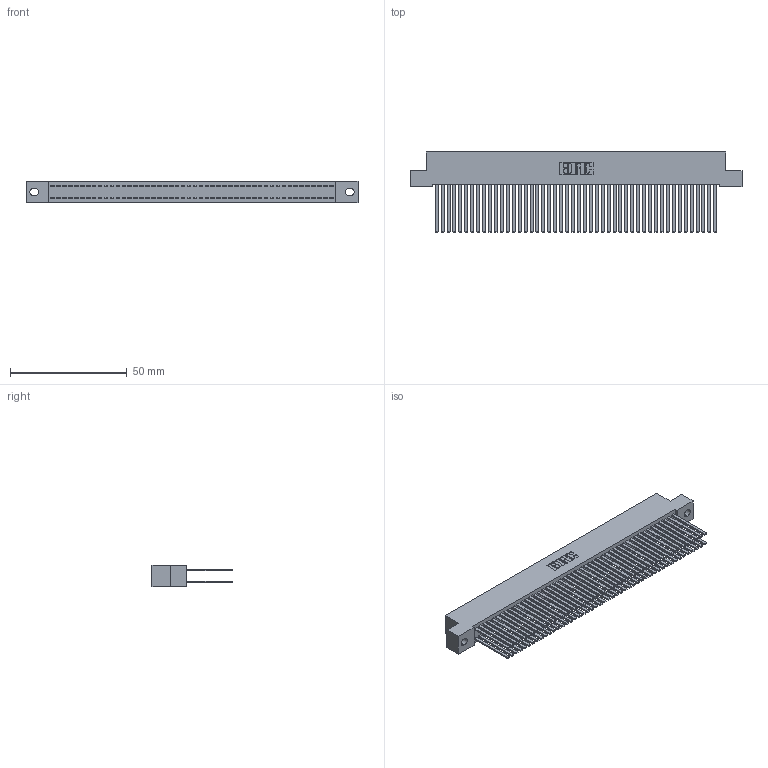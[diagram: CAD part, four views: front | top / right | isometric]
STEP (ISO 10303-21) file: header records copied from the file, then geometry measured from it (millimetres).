
FILE_DESCRIPTION (( 'STEP AP203' ), '1' );
FILE_NAME ('342-096-544-202.STEP', '2019-10-04T16:10:51', ( '' ), ( '' ), 'SwSTEP 2.0', 'SolidWorks 2016', '' );
FILE_SCHEMA (( 'CONFIG_CONTROL_DESIGN' ));
Length unit declared in the file: inch
Products named in the file (3): 342 Part_.128 Slot; 345-292-001_345-293-144; 342-096-544-202
Assembly tree (97 placements, depth 2):
  342-096-544-202
    342 Part_.128 Slot
    345-292-001_345-293-144  x96
Bounding box: 142.24 x 34.3 x 9.4 mm (x, y, z)
Volume: 14102.2 mm3; surface area: 26589.1 mm2
Topology: 97 solids, 97 shells, 4530 faces, 13463 edges, 8846 vertices
Faces by surface type: plane 3142, cylinder 1388
Entity records: 29923 total; most frequent: CARTESIAN_POINT 4950, ORIENTED_EDGE 4886, DIRECTION 4215, EDGE_CURVE 2443, LINE 2319, VECTOR 2319, VERTEX_POINT 1626, AXIS2_PLACEMENT_3D 948
